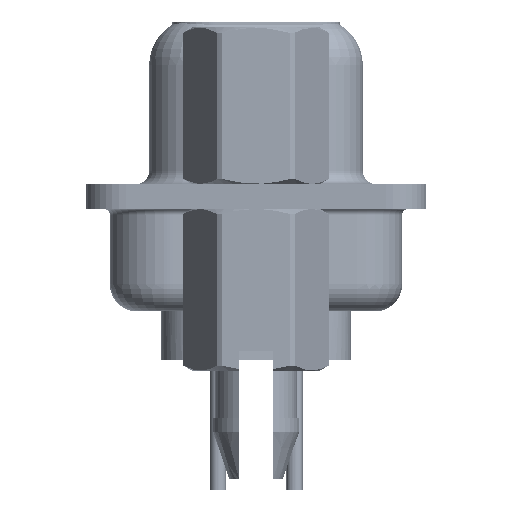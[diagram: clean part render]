
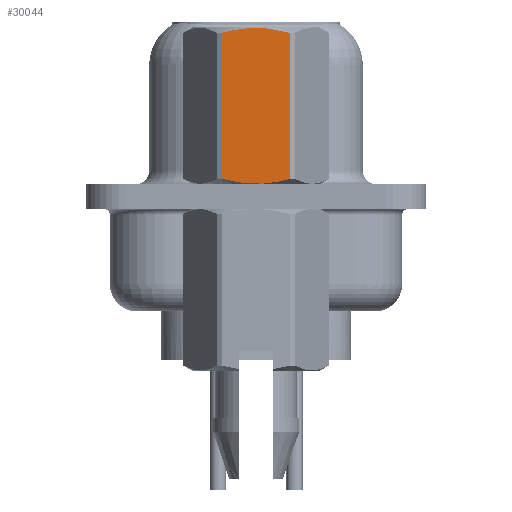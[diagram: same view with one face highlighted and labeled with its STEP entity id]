
A CAD part, left-side view. The second image highlights one B-rep face of the part: STEP entity #30044.
In plain terms, the highlighted planar face has unit normal (-1, 0, 0).
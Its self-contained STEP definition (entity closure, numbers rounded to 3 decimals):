
#48 = CARTESIAN_POINT ( 'NONE',  ( -2.381, -1.273, 0.652 ) ) ;
#258 = ORIENTED_EDGE ( 'NONE', *, *, #18772, .T. ) ;
#636 = EDGE_CURVE ( 'NONE', #14029, #26061, #30726, .T. ) ;
#1492 = CARTESIAN_POINT ( 'NONE',  ( -2.381, 1.065, 6.104 ) ) ;
#1818 = CARTESIAN_POINT ( 'NONE',  ( -2.381, -0.432, 6.215 ) ) ;
#1997 = CARTESIAN_POINT ( 'NONE',  ( -2.381, 0.215, 6.232 ) ) ;
#3925 = CARTESIAN_POINT ( 'NONE',  ( -2.381, -1.273, 6.048 ) ) ;
#4571 = CARTESIAN_POINT ( 'NONE',  ( -2.381, -0.215, 6.232 ) ) ;
#4758 = CARTESIAN_POINT ( 'NONE',  ( -2.381, 0.853, 6.151 ) ) ;
#5440 = VECTOR ( 'NONE', #17113, 1000. ) ;
#6042 = DIRECTION ( 'NONE',  ( 0., 0., -1. ) ) ;
#7967 = CARTESIAN_POINT ( 'NONE',  ( -2.381, 0.853, 0.549 ) ) ;
#8474 = EDGE_LOOP ( 'NONE', ( #32971, #31910, #258, #20299 ) ) ;
#9119 = LINE ( 'NONE', #29739, #22377 ) ;
#9196 = PLANE ( 'NONE',  #17288 ) ;
#9868 = CARTESIAN_POINT ( 'NONE',  ( -2.381, 1.273, 0.652 ) ) ;
#11975 = CARTESIAN_POINT ( 'NONE',  ( -2.381, 0.428, 6.215 ) ) ;
#12099 = CARTESIAN_POINT ( 'NONE',  ( -2.381, 1.375, -3.75 ) ) ;
#12613 = CARTESIAN_POINT ( 'NONE',  ( -2.381, -0.215, 0.468 ) ) ;
#13921 = B_SPLINE_CURVE_WITH_KNOTS ( 'NONE', 3,
 ( #9868, #28759, #7967, #23092, #21009, #12613, #33570, #18246, #28252, #48 ),
 .UNSPECIFIED., .F., .F.,
 ( 4, 2, 2, 2, 4 ),
 ( 0.003, 0.003, 0.004, 0.004, 0.005 ),
 .UNSPECIFIED. ) ;
#14029 = VERTEX_POINT ( 'NONE', #16844 ) ;
#14504 = DIRECTION ( 'NONE',  ( 0., -1., 0. ) ) ;
#15231 = CARTESIAN_POINT ( 'NONE',  ( -2.381, 1.273, 6.048 ) ) ;
#15305 = B_SPLINE_CURVE_WITH_KNOTS ( 'NONE', 3,
 ( #17779, #25538, #28297, #1818, #4571, #1997, #11975, #4758, #1492, #15231 ),
 .UNSPECIFIED., .F., .F.,
 ( 4, 2, 2, 2, 4 ),
 ( 0.001, 0.002, 0.002, 0.003, 0.004 ),
 .UNSPECIFIED. ) ;
#16328 = CARTESIAN_POINT ( 'NONE',  ( -2.381, 1.273, 6.048 ) ) ;
#16844 = CARTESIAN_POINT ( 'NONE',  ( -2.381, -1.273, 0.652 ) ) ;
#17041 = CARTESIAN_POINT ( 'NONE',  ( -2.381, 1.273, 0.652 ) ) ;
#17113 = DIRECTION ( 'NONE',  ( 0., 0., 1. ) ) ;
#17288 = AXIS2_PLACEMENT_3D ( 'NONE', #12099, #32920, #14504 ) ;
#17779 = CARTESIAN_POINT ( 'NONE',  ( -2.381, -1.273, 6.048 ) ) ;
#18246 = CARTESIAN_POINT ( 'NONE',  ( -2.381, -0.858, 0.55 ) ) ;
#18772 = EDGE_CURVE ( 'NONE', #26061, #29475, #15305, .T. ) ;
#19273 = EDGE_CURVE ( 'NONE', #29475, #22738, #9119, .T. ) ;
#20299 = ORIENTED_EDGE ( 'NONE', *, *, #19273, .T. ) ;
#21009 = CARTESIAN_POINT ( 'NONE',  ( -2.381, 0.215, 0.468 ) ) ;
#22377 = VECTOR ( 'NONE', #6042, 1000. ) ;
#22738 = VERTEX_POINT ( 'NONE', #17041 ) ;
#23092 = CARTESIAN_POINT ( 'NONE',  ( -2.381, 0.428, 0.485 ) ) ;
#23138 = CARTESIAN_POINT ( 'NONE',  ( -2.381, -1.273, 3.792 ) ) ;
#25538 = CARTESIAN_POINT ( 'NONE',  ( -2.381, -1.066, 6.104 ) ) ;
#26061 = VERTEX_POINT ( 'NONE', #3925 ) ;
#27404 = FACE_OUTER_BOUND ( 'NONE', #8474, .T. ) ;
#28252 = CARTESIAN_POINT ( 'NONE',  ( -2.381, -1.066, 0.596 ) ) ;
#28297 = CARTESIAN_POINT ( 'NONE',  ( -2.381, -0.858, 6.15 ) ) ;
#28748 = EDGE_CURVE ( 'NONE', #22738, #14029, #13921, .T. ) ;
#28759 = CARTESIAN_POINT ( 'NONE',  ( -2.381, 1.065, 0.596 ) ) ;
#29475 = VERTEX_POINT ( 'NONE', #16328 ) ;
#29739 = CARTESIAN_POINT ( 'NONE',  ( -2.381, 1.273, 3.792 ) ) ;
#30044 = ADVANCED_FACE ( 'NONE', ( #27404 ), #9196, .T. ) ;
#30726 = LINE ( 'NONE', #23138, #5440 ) ;
#31910 = ORIENTED_EDGE ( 'NONE', *, *, #636, .T. ) ;
#32920 = DIRECTION ( 'NONE',  ( -1., 0., 0. ) ) ;
#32971 = ORIENTED_EDGE ( 'NONE', *, *, #28748, .T. ) ;
#33570 = CARTESIAN_POINT ( 'NONE',  ( -2.381, -0.432, 0.485 ) ) ;
